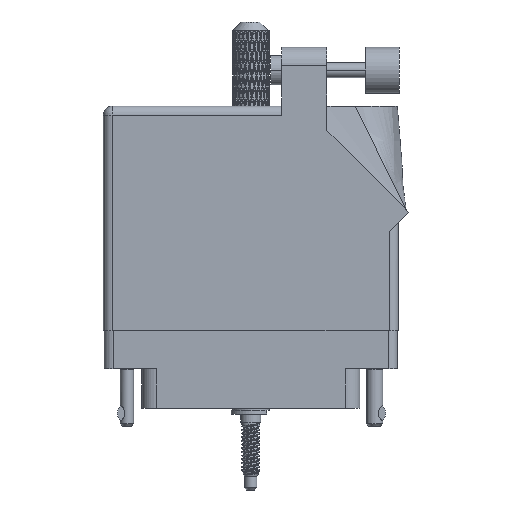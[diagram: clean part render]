
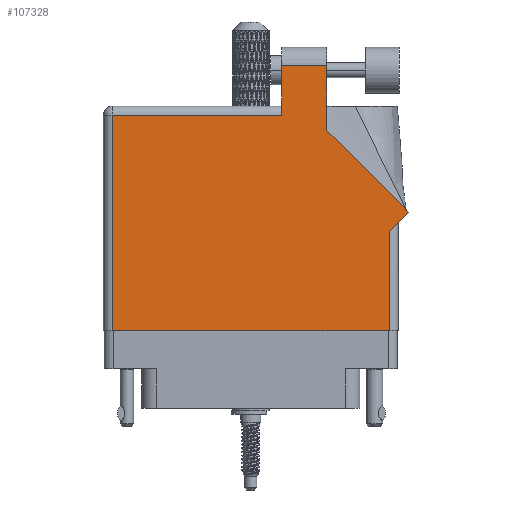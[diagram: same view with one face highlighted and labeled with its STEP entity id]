
A CAD part, front view. The second image highlights one B-rep face of the part: STEP entity #107328.
In plain terms, the highlighted face is planar.
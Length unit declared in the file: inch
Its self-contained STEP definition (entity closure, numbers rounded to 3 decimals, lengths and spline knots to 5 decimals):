
#680 = EDGE_LOOP ( 'NONE', ( #27315, #29527, #61885, #95818, #32538, #43608, #76177, #107396, #50746 ) ) ;
#1001 = CARTESIAN_POINT ( 'NONE',  ( 1.217, 1.53, 0. ) ) ;
#1598 = VECTOR ( 'NONE', #67788, 39.37008 ) ;
#1945 = VERTEX_POINT ( 'NONE', #70768 ) ;
#4454 = CARTESIAN_POINT ( 'NONE',  ( 0.062, 0., 0. ) ) ;
#5234 = DIRECTION ( 'NONE',  ( 0., -1., 0. ) ) ;
#10325 = CARTESIAN_POINT ( 'NONE',  ( 2.01, 0.737, 0. ) ) ;
#13760 = VECTOR ( 'NONE', #64481, 39.37008 ) ;
#14163 = VECTOR ( 'NONE', #5234, 39.37008 ) ;
#16016 = DIRECTION ( 'NONE',  ( -1., 0., 0. ) ) ;
#16065 = EDGE_CURVE ( 'NONE', #67427, #1945, #16940, .T. ) ;
#16214 = PLANE ( 'NONE',  #87106 ) ;
#16940 = LINE ( 'NONE', #4454, #14163 ) ;
#20023 = DIRECTION ( 'NONE',  ( -0.707, 0.707, 0. ) ) ;
#23027 = VERTEX_POINT ( 'NONE', #105692 ) ;
#24329 = EDGE_CURVE ( 'NONE', #46727, #74038, #39108, .T. ) ;
#26167 = CARTESIAN_POINT ( 'NONE',  ( 1.217, 1.468, 0. ) ) ;
#27315 = ORIENTED_EDGE ( 'NONE', *, *, #109727, .T. ) ;
#29527 = ORIENTED_EDGE ( 'NONE', *, *, #47392, .T. ) ;
#31071 = CARTESIAN_POINT ( 'NONE',  ( 0.062, 1.468, 0. ) ) ;
#31586 = LINE ( 'NONE', #68257, #81065 ) ;
#32538 = ORIENTED_EDGE ( 'NONE', *, *, #16065, .T. ) ;
#33676 = VECTOR ( 'NONE', #70592, 39.37008 ) ;
#34063 = VERTEX_POINT ( 'NONE', #106609 ) ;
#34094 = CARTESIAN_POINT ( 'NONE',  ( 1.524, 1.36442, 0. ) ) ;
#35553 = CARTESIAN_POINT ( 'NONE',  ( 2.08071, 0.80771, 0. ) ) ;
#36053 = VECTOR ( 'NONE', #84681, 39.37008 ) ;
#39108 = LINE ( 'NONE', #1001, #33676 ) ;
#39672 = LINE ( 'NONE', #68698, #72672 ) ;
#40048 = VECTOR ( 'NONE', #20023, 39.37008 ) ;
#40090 = LINE ( 'NONE', #67409, #1598 ) ;
#40126 = VECTOR ( 'NONE', #94719, 39.37008 ) ;
#41544 = FACE_OUTER_BOUND ( 'NONE', #680, .T. ) ;
#42293 = EDGE_CURVE ( 'NONE', #1945, #34063, #108962, .T. ) ;
#43608 = ORIENTED_EDGE ( 'NONE', *, *, #42293, .T. ) ;
#46727 = VERTEX_POINT ( 'NONE', #54117 ) ;
#47392 = EDGE_CURVE ( 'NONE', #53481, #46727, #40090, .T. ) ;
#50746 = ORIENTED_EDGE ( 'NONE', *, *, #52779, .T. ) ;
#52779 = EDGE_CURVE ( 'NONE', #63960, #90037, #81291, .T. ) ;
#53481 = VERTEX_POINT ( 'NONE', #59426 ) ;
#54117 = CARTESIAN_POINT ( 'NONE',  ( 1.217, 1.805, 0. ) ) ;
#59426 = CARTESIAN_POINT ( 'NONE',  ( 1.524, 1.805, 0. ) ) ;
#60479 = LINE ( 'NONE', #10325, #13760 ) ;
#61885 = ORIENTED_EDGE ( 'NONE', *, *, #24329, .T. ) ;
#62124 = LINE ( 'NONE', #102369, #36053 ) ;
#63960 = VERTEX_POINT ( 'NONE', #35553 ) ;
#64293 = EDGE_CURVE ( 'NONE', #34063, #23027, #62124, .T. ) ;
#64481 = DIRECTION ( 'NONE',  ( 0.707, 0.707, 0. ) ) ;
#67409 = CARTESIAN_POINT ( 'NONE',  ( 1.217, 1.805, 0. ) ) ;
#67427 = VERTEX_POINT ( 'NONE', #31071 ) ;
#67788 = DIRECTION ( 'NONE',  ( -1., 0., 0. ) ) ;
#68257 = CARTESIAN_POINT ( 'NONE',  ( 1.524, 1.36442, 0. ) ) ;
#68698 = CARTESIAN_POINT ( 'NONE',  ( 0., 1.468, 0. ) ) ;
#70592 = DIRECTION ( 'NONE',  ( 0., -1., 0. ) ) ;
#70768 = CARTESIAN_POINT ( 'NONE',  ( 0.062, 0., 0. ) ) ;
#72672 = VECTOR ( 'NONE', #16016, 39.37008 ) ;
#72725 = CARTESIAN_POINT ( 'NONE',  ( 2.08071, 0.80771, 0. ) ) ;
#74038 = VERTEX_POINT ( 'NONE', #26167 ) ;
#75915 = CARTESIAN_POINT ( 'NONE',  ( 0., 0., 0. ) ) ;
#76177 = ORIENTED_EDGE ( 'NONE', *, *, #64293, .T. ) ;
#76974 = CARTESIAN_POINT ( 'NONE',  ( 0., 1.53, 0. ) ) ;
#81065 = VECTOR ( 'NONE', #85025, 39.37008 ) ;
#81291 = LINE ( 'NONE', #72725, #40048 ) ;
#84681 = DIRECTION ( 'NONE',  ( 0., 1., 0. ) ) ;
#85025 = DIRECTION ( 'NONE',  ( 0., 1., 0. ) ) ;
#85109 = EDGE_CURVE ( 'NONE', #23027, #63960, #60479, .T. ) ;
#86448 = EDGE_CURVE ( 'NONE', #74038, #67427, #39672, .T. ) ;
#87106 = AXIS2_PLACEMENT_3D ( 'NONE', #76974, #103891, #95457 ) ;
#90037 = VERTEX_POINT ( 'NONE', #34094 ) ;
#94719 = DIRECTION ( 'NONE',  ( 1., 0., 0. ) ) ;
#95457 = DIRECTION ( 'NONE',  ( -1., 0., 0. ) ) ;
#95818 = ORIENTED_EDGE ( 'NONE', *, *, #86448, .T. ) ;
#102369 = CARTESIAN_POINT ( 'NONE',  ( 1.948, 0.737, 0. ) ) ;
#103891 = DIRECTION ( 'NONE',  ( 0., 0., -1. ) ) ;
#105692 = CARTESIAN_POINT ( 'NONE',  ( 1.948, 0.675, 0. ) ) ;
#106609 = CARTESIAN_POINT ( 'NONE',  ( 1.948, 0., 0. ) ) ;
#107328 = ADVANCED_FACE ( 'NONE', ( #41544 ), #16214, .F. ) ;
#107396 = ORIENTED_EDGE ( 'NONE', *, *, #85109, .T. ) ;
#108962 = LINE ( 'NONE', #75915, #40126 ) ;
#109727 = EDGE_CURVE ( 'NONE', #90037, #53481, #31586, .T. ) ;
